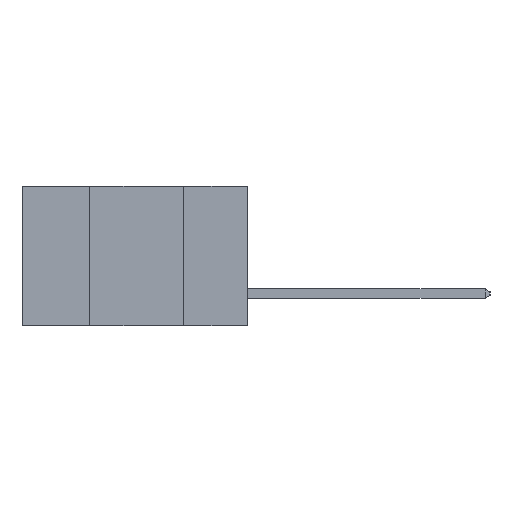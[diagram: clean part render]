
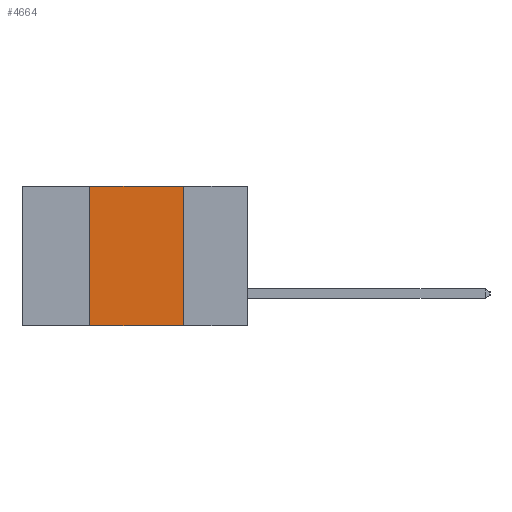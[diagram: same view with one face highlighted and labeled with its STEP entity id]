
A CAD part, left-side view. The second image highlights one B-rep face of the part: STEP entity #4664.
In plain terms, the highlighted planar face has unit normal (-1, 0, 0).
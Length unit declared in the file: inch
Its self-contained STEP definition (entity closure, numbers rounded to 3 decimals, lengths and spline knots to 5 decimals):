
#5 = LINE ( 'NONE', #7706, #13400 ) ;
#224 = EDGE_CURVE ( 'NONE', #5547, #15053, #8418, .T. ) ;
#461 = DIRECTION ( 'NONE',  ( 0., 0., -1. ) ) ;
#523 = DIRECTION ( 'NONE',  ( 1., 0., 0. ) ) ;
#704 = PLANE ( 'NONE',  #5398 ) ;
#1169 = CARTESIAN_POINT ( 'NONE',  ( 0., 0.6, 0. ) ) ;
#1319 = VECTOR ( 'NONE', #9921, 39.37008 ) ;
#1625 = FACE_OUTER_BOUND ( 'NONE', #16234, .T. ) ;
#2008 = ORIENTED_EDGE ( 'NONE', *, *, #224, .F. ) ;
#2663 = CARTESIAN_POINT ( 'NONE',  ( 0., 0.17, 0. ) ) ;
#2738 = VERTEX_POINT ( 'NONE', #16491 ) ;
#3984 = LINE ( 'NONE', #16495, #7525 ) ;
#4664 = ADVANCED_FACE ( 'NONE', ( #1625 ), #704, .F. ) ;
#5398 = AXIS2_PLACEMENT_3D ( 'NONE', #1169, #523, #461 ) ;
#5547 = VERTEX_POINT ( 'NONE', #15828 ) ;
#7146 = LINE ( 'NONE', #7895, #14242 ) ;
#7181 = VERTEX_POINT ( 'NONE', #2663 ) ;
#7305 = DIRECTION ( 'NONE',  ( 0., -1., 0. ) ) ;
#7525 = VECTOR ( 'NONE', #7305, 39.37008 ) ;
#7706 = CARTESIAN_POINT ( 'NONE',  ( 0., 0.17, -0.37 ) ) ;
#7820 = DIRECTION ( 'NONE',  ( 0., 0., -1. ) ) ;
#7834 = ORIENTED_EDGE ( 'NONE', *, *, #9490, .T. ) ;
#7895 = CARTESIAN_POINT ( 'NONE',  ( 0., 0.6, -0.37 ) ) ;
#7942 = DIRECTION ( 'NONE',  ( 0., -1., 0. ) ) ;
#8418 = LINE ( 'NONE', #11950, #1319 ) ;
#9490 = EDGE_CURVE ( 'NONE', #5547, #2738, #7146, .T. ) ;
#9512 = EDGE_CURVE ( 'NONE', #7181, #2738, #5, .T. ) ;
#9921 = DIRECTION ( 'NONE',  ( 0., 0., 1. ) ) ;
#10810 = ORIENTED_EDGE ( 'NONE', *, *, #9512, .F. ) ;
#11193 = ORIENTED_EDGE ( 'NONE', *, *, #12194, .F. ) ;
#11950 = CARTESIAN_POINT ( 'NONE',  ( 0., 0.42, -0.37 ) ) ;
#12194 = EDGE_CURVE ( 'NONE', #15053, #7181, #3984, .T. ) ;
#13400 = VECTOR ( 'NONE', #7820, 39.37008 ) ;
#14242 = VECTOR ( 'NONE', #7942, 39.37008 ) ;
#15053 = VERTEX_POINT ( 'NONE', #16812 ) ;
#15828 = CARTESIAN_POINT ( 'NONE',  ( 0., 0.42, -0.37 ) ) ;
#16234 = EDGE_LOOP ( 'NONE', ( #10810, #11193, #2008, #7834 ) ) ;
#16491 = CARTESIAN_POINT ( 'NONE',  ( 0., 0.17, -0.37 ) ) ;
#16495 = CARTESIAN_POINT ( 'NONE',  ( 0., 0.6, 0. ) ) ;
#16812 = CARTESIAN_POINT ( 'NONE',  ( 0., 0.42, 0. ) ) ;
